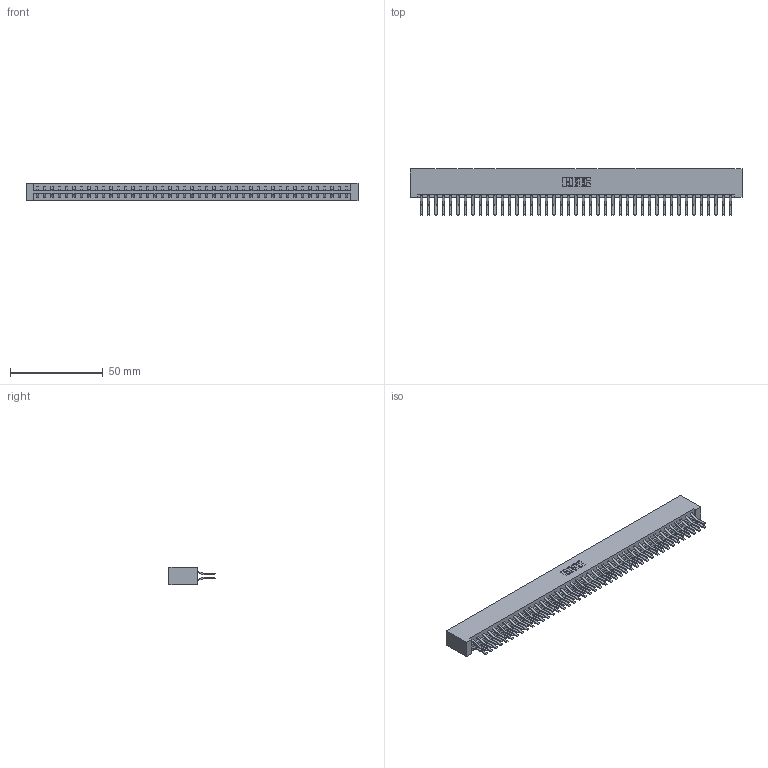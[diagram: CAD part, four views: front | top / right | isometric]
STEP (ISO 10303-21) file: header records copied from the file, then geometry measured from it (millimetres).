
FILE_DESCRIPTION (( 'STEP AP203' ), '1' );
FILE_NAME ('833-086-560-201.STEP', '2020-06-06T04:23:18', ( '' ), ( '' ), 'SwSTEP 2.0', 'SolidWorks 2020', '' );
FILE_SCHEMA (( 'CONFIG_CONTROL_DESIGN' ));
Length unit declared in the file: inch
Products named in the file (3): 345-292-001_560 Tail; 833 Part_Lugless; 833-086-560-201
Assembly tree (87 placements, depth 2):
  833-086-560-201
    833 Part_Lugless
    345-292-001_560 Tail  x86
Bounding box: 178.64 x 24.78 x 9.4 mm (x, y, z)
Volume: 19443.2 mm3; surface area: 24629.9 mm2
Topology: 87 solids, 87 shells, 4750 faces, 14133 edges, 9306 vertices
Faces by surface type: plane 3162, cylinder 1588
Entity records: 27345 total; most frequent: CARTESIAN_POINT 4530, ORIENTED_EDGE 4466, DIRECTION 3865, EDGE_CURVE 2233, VECTOR 2109, LINE 2109, VERTEX_POINT 1486, AXIS2_PLACEMENT_3D 878
